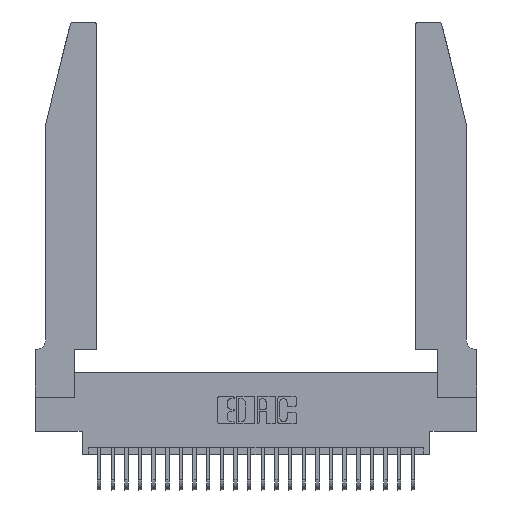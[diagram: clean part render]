
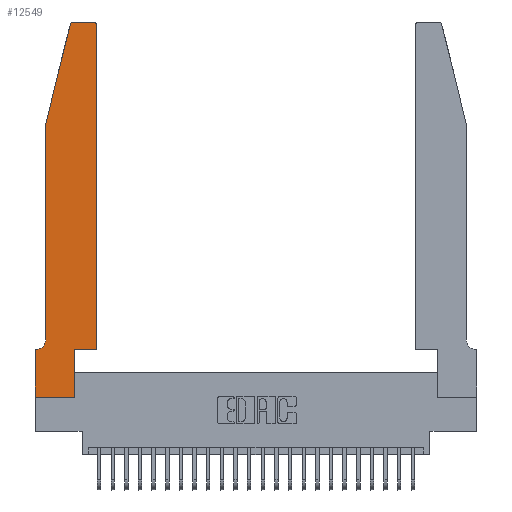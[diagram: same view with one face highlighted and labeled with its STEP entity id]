
A CAD part, top view. The second image highlights one B-rep face of the part: STEP entity #12549.
In plain terms, the highlighted planar face has unit normal (0, 0, 1).
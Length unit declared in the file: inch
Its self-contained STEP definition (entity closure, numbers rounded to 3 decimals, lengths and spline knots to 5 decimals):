
#195 = EDGE_CURVE ( 'NONE', #16119, #8724, #27057, .T. ) ;
#891 = EDGE_LOOP ( 'NONE', ( #24903, #8952, #12495, #18414, #5880, #11575, #18866, #10763, #27811, #17749, #7328, #20262 ) ) ;
#1301 = VERTEX_POINT ( 'NONE', #4966 ) ;
#1317 = EDGE_CURVE ( 'NONE', #8724, #2320, #20226, .T. ) ;
#1518 = CARTESIAN_POINT ( 'NONE',  ( 0., 0., 0.37 ) ) ;
#2105 = CARTESIAN_POINT ( 'NONE',  ( 0., 0., 0.37 ) ) ;
#2320 = VERTEX_POINT ( 'NONE', #8519 ) ;
#2829 = CIRCLE ( 'NONE', #20446, 0.07 ) ;
#3282 = AXIS2_PLACEMENT_3D ( 'NONE', #12412, #27018, #14570 ) ;
#3501 = EDGE_CURVE ( 'NONE', #6381, #16119, #23920, .T. ) ;
#3745 = DIRECTION ( 'NONE',  ( 1., 0., 0. ) ) ;
#3916 = EDGE_CURVE ( 'NONE', #2320, #12479, #14494, .T. ) ;
#3967 = CARTESIAN_POINT ( 'NONE',  ( 0.2865, 0., 0.37 ) ) ;
#4127 = VECTOR ( 'NONE', #11713, 39.37008 ) ;
#4256 = CARTESIAN_POINT ( 'NONE',  ( 0.284, 2.75, 0.37 ) ) ;
#4509 = DIRECTION ( 'NONE',  ( 1., 0., 0. ) ) ;
#4545 = CARTESIAN_POINT ( 'NONE',  ( 0.2605, 2.75, 0.37 ) ) ;
#4554 = CARTESIAN_POINT ( 'NONE',  ( 0.4505, 0.35, 0.37 ) ) ;
#4966 = CARTESIAN_POINT ( 'NONE',  ( 0.25487, 2.72718, 0.37 ) ) ;
#5239 = VECTOR ( 'NONE', #21583, 39.37008 ) ;
#5880 = ORIENTED_EDGE ( 'NONE', *, *, #18621, .T. ) ;
#5954 = LINE ( 'NONE', #2105, #5239 ) ;
#6027 = VERTEX_POINT ( 'NONE', #24154 ) ;
#6360 = VECTOR ( 'NONE', #18966, 39.37008 ) ;
#6381 = VERTEX_POINT ( 'NONE', #13185 ) ;
#6826 = DIRECTION ( 'NONE',  ( 0., 1., 0. ) ) ;
#7328 = ORIENTED_EDGE ( 'NONE', *, *, #3916, .T. ) ;
#7738 = VECTOR ( 'NONE', #9890, 39.37008 ) ;
#8160 = VECTOR ( 'NONE', #4509, 39.37008 ) ;
#8201 = CIRCLE ( 'NONE', #19063, 0.03 ) ;
#8275 = CARTESIAN_POINT ( 'NONE',  ( 0.0755, 2., 0.37 ) ) ;
#8519 = CARTESIAN_POINT ( 'NONE',  ( 0.4505, 0.35, 0.37 ) ) ;
#8724 = VERTEX_POINT ( 'NONE', #15389 ) ;
#8952 = ORIENTED_EDGE ( 'NONE', *, *, #27111, .T. ) ;
#8958 = LINE ( 'NONE', #14607, #25803 ) ;
#9255 = VERTEX_POINT ( 'NONE', #21106 ) ;
#9890 = DIRECTION ( 'NONE',  ( 0., -1., 0. ) ) ;
#10009 = VERTEX_POINT ( 'NONE', #4256 ) ;
#10292 = VECTOR ( 'NONE', #6826, 39.37008 ) ;
#10477 = DIRECTION ( 'NONE',  ( 0., 0., 1. ) ) ;
#10638 = CARTESIAN_POINT ( 'NONE',  ( 0.0055, 0.42, 0.37 ) ) ;
#10664 = CARTESIAN_POINT ( 'NONE',  ( 0.4505, 2.72, 0.37 ) ) ;
#10763 = ORIENTED_EDGE ( 'NONE', *, *, #3501, .T. ) ;
#11058 = EDGE_CURVE ( 'NONE', #20272, #6027, #19167, .T. ) ;
#11575 = ORIENTED_EDGE ( 'NONE', *, *, #13862, .T. ) ;
#11713 = DIRECTION ( 'NONE',  ( 0., 1., 0. ) ) ;
#12412 = CARTESIAN_POINT ( 'NONE',  ( 0.284, 2.72, 0.37 ) ) ;
#12438 = VERTEX_POINT ( 'NONE', #25290 ) ;
#12457 = DIRECTION ( 'NONE',  ( -1., 0., 0. ) ) ;
#12479 = VERTEX_POINT ( 'NONE', #10664 ) ;
#12495 = ORIENTED_EDGE ( 'NONE', *, *, #18042, .T. ) ;
#12549 = ADVANCED_FACE ( 'NONE', ( #16460 ), #25564, .T. ) ;
#12864 = DIRECTION ( 'NONE',  ( -1., 0., 0. ) ) ;
#13173 = DIRECTION ( 'NONE',  ( 0., 0., 1. ) ) ;
#13185 = CARTESIAN_POINT ( 'NONE',  ( 0., 0., 0.37 ) ) ;
#13733 = CARTESIAN_POINT ( 'NONE',  ( 0.0055, 0.35, 0.37 ) ) ;
#13835 = CARTESIAN_POINT ( 'NONE',  ( 0.2865, 0.35, 0.37 ) ) ;
#13862 = EDGE_CURVE ( 'NONE', #25714, #12438, #8958, .T. ) ;
#14494 = LINE ( 'NONE', #24283, #4127 ) ;
#14570 = DIRECTION ( 'NONE',  ( 1., 0., 0. ) ) ;
#14607 = CARTESIAN_POINT ( 'NONE',  ( 0.0755, 0.35, 0.37 ) ) ;
#15389 = CARTESIAN_POINT ( 'NONE',  ( 0.2865, 0.35, 0.37 ) ) ;
#16119 = VERTEX_POINT ( 'NONE', #3967 ) ;
#16273 = EDGE_CURVE ( 'NONE', #9255, #10009, #18641, .T. ) ;
#16460 = FACE_OUTER_BOUND ( 'NONE', #891, .T. ) ;
#17433 = CIRCLE ( 'NONE', #3282, 0.03 ) ;
#17749 = ORIENTED_EDGE ( 'NONE', *, *, #1317, .T. ) ;
#17877 = LINE ( 'NONE', #8275, #6360 ) ;
#17972 = VECTOR ( 'NONE', #25839, 39.37008 ) ;
#18042 = EDGE_CURVE ( 'NONE', #1301, #20272, #17877, .T. ) ;
#18414 = ORIENTED_EDGE ( 'NONE', *, *, #11058, .T. ) ;
#18621 = EDGE_CURVE ( 'NONE', #6027, #25714, #2829, .T. ) ;
#18641 = LINE ( 'NONE', #4545, #17972 ) ;
#18866 = ORIENTED_EDGE ( 'NONE', *, *, #25534, .T. ) ;
#18966 = DIRECTION ( 'NONE',  ( -0.239, -0.971, 0. ) ) ;
#19063 = AXIS2_PLACEMENT_3D ( 'NONE', #23130, #10477, #25201 ) ;
#19167 = LINE ( 'NONE', #20504, #7738 ) ;
#20226 = LINE ( 'NONE', #4554, #8160 ) ;
#20262 = ORIENTED_EDGE ( 'NONE', *, *, #23146, .T. ) ;
#20272 = VERTEX_POINT ( 'NONE', #25401 ) ;
#20446 = AXIS2_PLACEMENT_3D ( 'NONE', #10638, #25362, #12864 ) ;
#20504 = CARTESIAN_POINT ( 'NONE',  ( 0.0755, 2., 0.37 ) ) ;
#21106 = CARTESIAN_POINT ( 'NONE',  ( 0.4205, 2.75, 0.37 ) ) ;
#21583 = DIRECTION ( 'NONE',  ( 0., -1., 0. ) ) ;
#23130 = CARTESIAN_POINT ( 'NONE',  ( 0.4205, 2.72, 0.37 ) ) ;
#23146 = EDGE_CURVE ( 'NONE', #12479, #9255, #8201, .T. ) ;
#23263 = VECTOR ( 'NONE', #3745, 39.37008 ) ;
#23568 = CARTESIAN_POINT ( 'NONE',  ( 0., 0.35, 0.37 ) ) ;
#23920 = LINE ( 'NONE', #1518, #23263 ) ;
#24154 = CARTESIAN_POINT ( 'NONE',  ( 0.0755, 0.42, 0.37 ) ) ;
#24283 = CARTESIAN_POINT ( 'NONE',  ( 0.4505, 0.35, 0.37 ) ) ;
#24903 = ORIENTED_EDGE ( 'NONE', *, *, #16273, .T. ) ;
#25201 = DIRECTION ( 'NONE',  ( 1., 0., 0. ) ) ;
#25290 = CARTESIAN_POINT ( 'NONE',  ( 0., 0.35, 0.37 ) ) ;
#25362 = DIRECTION ( 'NONE',  ( 0., 0., -1. ) ) ;
#25401 = CARTESIAN_POINT ( 'NONE',  ( 0.0755, 2., 0.37 ) ) ;
#25534 = EDGE_CURVE ( 'NONE', #12438, #6381, #5954, .T. ) ;
#25564 = PLANE ( 'NONE',  #26548 ) ;
#25714 = VERTEX_POINT ( 'NONE', #13733 ) ;
#25803 = VECTOR ( 'NONE', #12457, 39.37008 ) ;
#25839 = DIRECTION ( 'NONE',  ( -1., 0., 0. ) ) ;
#26548 = AXIS2_PLACEMENT_3D ( 'NONE', #23568, #13173, #27723 ) ;
#27018 = DIRECTION ( 'NONE',  ( 0., 0., 1. ) ) ;
#27057 = LINE ( 'NONE', #13835, #10292 ) ;
#27111 = EDGE_CURVE ( 'NONE', #10009, #1301, #17433, .T. ) ;
#27723 = DIRECTION ( 'NONE',  ( 1., 0., 0. ) ) ;
#27811 = ORIENTED_EDGE ( 'NONE', *, *, #195, .T. ) ;
